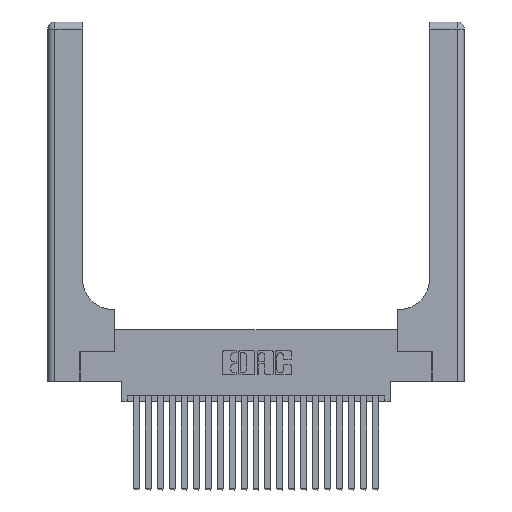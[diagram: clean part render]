
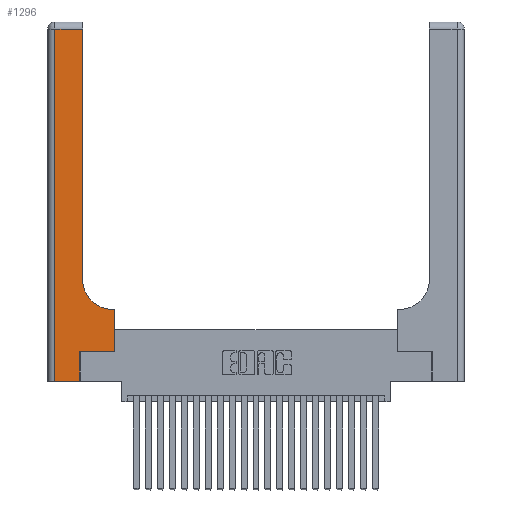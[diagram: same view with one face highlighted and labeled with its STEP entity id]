
A CAD part, top view. The second image highlights one B-rep face of the part: STEP entity #1296.
In plain terms, the highlighted planar face has unit normal (0, 0, 1).
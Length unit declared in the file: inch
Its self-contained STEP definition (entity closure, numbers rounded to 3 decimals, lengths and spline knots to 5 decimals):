
#900 = CARTESIAN_POINT ( 'NONE',  ( 0.2915, 0.6, 0.37 ) ) ;
#1171 = CARTESIAN_POINT ( 'NONE',  ( 0.2915, 0.85, 0.37 ) ) ;
#1252 = CARTESIAN_POINT ( 'NONE',  ( 0.5415, 0.6, 0.37 ) ) ;
#1285 = CARTESIAN_POINT ( 'NONE',  ( 0.06, 3., 0.37 ) ) ;
#1296 = ADVANCED_FACE ( 'NONE', ( #11819 ), #4277, .F. ) ;
#1382 = EDGE_CURVE ( 'NONE', #12263, #19805, #11232, .T. ) ;
#1766 = CARTESIAN_POINT ( 'NONE',  ( 0.2915, 2.94, 0.37 ) ) ;
#2421 = DIRECTION ( 'NONE',  ( 0., 0., -1. ) ) ;
#2624 = DIRECTION ( 'NONE',  ( 1., 0., 0. ) ) ;
#3566 = VECTOR ( 'NONE', #11378, 39.37008 ) ;
#3620 = EDGE_LOOP ( 'NONE', ( #17400, #20395, #10887, #18619, #22815, #5073, #13726, #5422, #21818 ) ) ;
#3897 = CARTESIAN_POINT ( 'NONE',  ( 0.5585, 0.25, 0.37 ) ) ;
#4020 = VERTEX_POINT ( 'NONE', #1766 ) ;
#4161 = CARTESIAN_POINT ( 'NONE',  ( 0.269, 0.25, 0.37 ) ) ;
#4277 = PLANE ( 'NONE',  #16254 ) ;
#4756 = LINE ( 'NONE', #16616, #24164 ) ;
#4764 = DIRECTION ( 'NONE',  ( -1., 0., 0. ) ) ;
#4930 = VERTEX_POINT ( 'NONE', #5001 ) ;
#5001 = CARTESIAN_POINT ( 'NONE',  ( 0.269, 0.25, 0.37 ) ) ;
#5073 = ORIENTED_EDGE ( 'NONE', *, *, #16097, .T. ) ;
#5422 = ORIENTED_EDGE ( 'NONE', *, *, #1382, .T. ) ;
#5744 = CARTESIAN_POINT ( 'NONE',  ( 0.5585, 0.6, 0.37 ) ) ;
#5804 = VERTEX_POINT ( 'NONE', #14960 ) ;
#6124 = DIRECTION ( 'NONE',  ( 0., 0., -1. ) ) ;
#8101 = CARTESIAN_POINT ( 'NONE',  ( 0., 3., 0.37 ) ) ;
#8661 = AXIS2_PLACEMENT_3D ( 'NONE', #17367, #6124, #19221 ) ;
#9239 = VERTEX_POINT ( 'NONE', #22490 ) ;
#9610 = DIRECTION ( 'NONE',  ( 0., 1., 0. ) ) ;
#9804 = LINE ( 'NONE', #15144, #3566 ) ;
#10231 = VERTEX_POINT ( 'NONE', #1171 ) ;
#10253 = VECTOR ( 'NONE', #12699, 39.37008 ) ;
#10366 = LINE ( 'NONE', #15878, #15367 ) ;
#10887 = ORIENTED_EDGE ( 'NONE', *, *, #13010, .T. ) ;
#11232 = LINE ( 'NONE', #900, #20559 ) ;
#11378 = DIRECTION ( 'NONE',  ( -1., 0., 0. ) ) ;
#11819 = FACE_OUTER_BOUND ( 'NONE', #3620, .T. ) ;
#12246 = CARTESIAN_POINT ( 'NONE',  ( 0.5585, 0.25, 0.37 ) ) ;
#12263 = VERTEX_POINT ( 'NONE', #5744 ) ;
#12699 = DIRECTION ( 'NONE',  ( 0., -1., 0. ) ) ;
#12708 = LINE ( 'NONE', #3897, #20848 ) ;
#13010 = EDGE_CURVE ( 'NONE', #15803, #9239, #16429, .T. ) ;
#13164 = DIRECTION ( 'NONE',  ( 0., 1., 0. ) ) ;
#13726 = ORIENTED_EDGE ( 'NONE', *, *, #16652, .T. ) ;
#14432 = EDGE_CURVE ( 'NONE', #19805, #10231, #18373, .T. ) ;
#14675 = CARTESIAN_POINT ( 'NONE',  ( 0.06, 2.94, 0.37 ) ) ;
#14960 = CARTESIAN_POINT ( 'NONE',  ( 0.269, 0., 0.37 ) ) ;
#15144 = CARTESIAN_POINT ( 'NONE',  ( 0., 2.94, 0.37 ) ) ;
#15367 = VECTOR ( 'NONE', #2624, 39.37008 ) ;
#15673 = DIRECTION ( 'NONE',  ( -1., 0., 0. ) ) ;
#15803 = VERTEX_POINT ( 'NONE', #14675 ) ;
#15878 = CARTESIAN_POINT ( 'NONE',  ( 0., 0., 0.37 ) ) ;
#16097 = EDGE_CURVE ( 'NONE', #4930, #16920, #20589, .T. ) ;
#16254 = AXIS2_PLACEMENT_3D ( 'NONE', #8101, #2421, #15673 ) ;
#16261 = EDGE_CURVE ( 'NONE', #9239, #5804, #10366, .T. ) ;
#16429 = LINE ( 'NONE', #1285, #10253 ) ;
#16616 = CARTESIAN_POINT ( 'NONE',  ( 0.2915, 3., 0.37 ) ) ;
#16652 = EDGE_CURVE ( 'NONE', #16920, #12263, #12708, .T. ) ;
#16920 = VERTEX_POINT ( 'NONE', #12246 ) ;
#17367 = CARTESIAN_POINT ( 'NONE',  ( 0.5415, 0.85, 0.37 ) ) ;
#17400 = ORIENTED_EDGE ( 'NONE', *, *, #21077, .T. ) ;
#17804 = VECTOR ( 'NONE', #13164, 39.37008 ) ;
#18373 = CIRCLE ( 'NONE', #8661, 0.25 ) ;
#18619 = ORIENTED_EDGE ( 'NONE', *, *, #16261, .T. ) ;
#19221 = DIRECTION ( 'NONE',  ( 1., 0., 0. ) ) ;
#19527 = EDGE_CURVE ( 'NONE', #5804, #4930, #22766, .T. ) ;
#19805 = VERTEX_POINT ( 'NONE', #1252 ) ;
#20325 = DIRECTION ( 'NONE',  ( 0., 1., 0. ) ) ;
#20395 = ORIENTED_EDGE ( 'NONE', *, *, #22559, .T. ) ;
#20559 = VECTOR ( 'NONE', #4764, 39.37008 ) ;
#20589 = LINE ( 'NONE', #4161, #21160 ) ;
#20848 = VECTOR ( 'NONE', #9610, 39.37008 ) ;
#21077 = EDGE_CURVE ( 'NONE', #10231, #4020, #4756, .T. ) ;
#21160 = VECTOR ( 'NONE', #22891, 39.37008 ) ;
#21818 = ORIENTED_EDGE ( 'NONE', *, *, #14432, .T. ) ;
#22451 = CARTESIAN_POINT ( 'NONE',  ( 0.269, 0., 0.37 ) ) ;
#22490 = CARTESIAN_POINT ( 'NONE',  ( 0.06, 0., 0.37 ) ) ;
#22559 = EDGE_CURVE ( 'NONE', #4020, #15803, #9804, .T. ) ;
#22766 = LINE ( 'NONE', #22451, #17804 ) ;
#22815 = ORIENTED_EDGE ( 'NONE', *, *, #19527, .T. ) ;
#22891 = DIRECTION ( 'NONE',  ( 1., 0., 0. ) ) ;
#24164 = VECTOR ( 'NONE', #20325, 39.37008 ) ;
